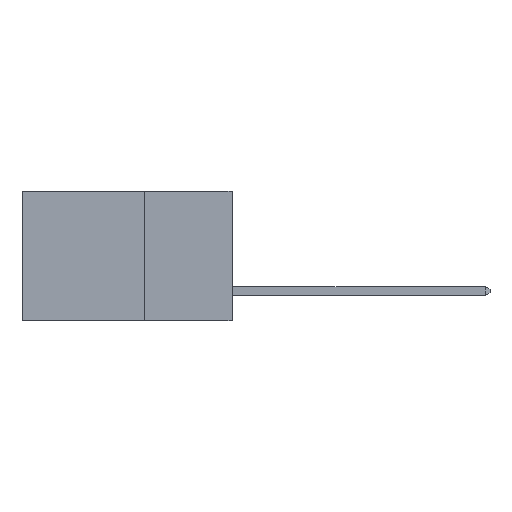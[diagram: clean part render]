
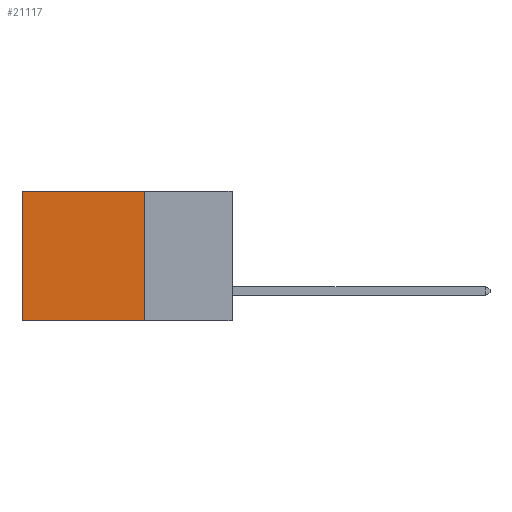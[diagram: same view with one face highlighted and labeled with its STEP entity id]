
A CAD part, left-side view. The second image highlights one B-rep face of the part: STEP entity #21117.
In plain terms, the highlighted planar face has unit normal (-1, 0, 0).
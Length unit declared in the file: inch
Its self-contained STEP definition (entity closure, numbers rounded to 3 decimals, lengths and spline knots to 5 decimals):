
#407 = VECTOR ( 'NONE', #17627, 39.37008 ) ;
#603 = DIRECTION ( 'NONE',  ( 0., 1., 0. ) ) ;
#798 = DIRECTION ( 'NONE',  ( 1., 0., 0. ) ) ;
#2346 = CARTESIAN_POINT ( 'NONE',  ( 0.2875, 0.25, 0. ) ) ;
#2445 = EDGE_CURVE ( 'NONE', #16082, #22579, #5867, .T. ) ;
#2901 = CARTESIAN_POINT ( 'NONE',  ( 0.2875, 0.6, 0. ) ) ;
#4182 = CARTESIAN_POINT ( 'NONE',  ( 0.2875, 0.6, -0.37 ) ) ;
#5738 = EDGE_CURVE ( 'NONE', #22579, #18657, #14520, .T. ) ;
#5787 = VECTOR ( 'NONE', #9420, 39.37008 ) ;
#5867 = LINE ( 'NONE', #2346, #14630 ) ;
#8053 = ORIENTED_EDGE ( 'NONE', *, *, #15060, .T. ) ;
#8632 = LINE ( 'NONE', #11225, #17955 ) ;
#9420 = DIRECTION ( 'NONE',  ( 0., 0., -1. ) ) ;
#10304 = CARTESIAN_POINT ( 'NONE',  ( 0.2875, 0.25, 0. ) ) ;
#10368 = ORIENTED_EDGE ( 'NONE', *, *, #19866, .T. ) ;
#10965 = VERTEX_POINT ( 'NONE', #2901 ) ;
#11225 = CARTESIAN_POINT ( 'NONE',  ( 0.2875, 0.25, 0. ) ) ;
#11958 = CARTESIAN_POINT ( 'NONE',  ( 0.2875, 0.25, -0.37 ) ) ;
#13042 = CARTESIAN_POINT ( 'NONE',  ( 0.2875, 0.6, 0. ) ) ;
#13188 = DIRECTION ( 'NONE',  ( 0., 0., -1. ) ) ;
#13786 = FACE_OUTER_BOUND ( 'NONE', #16669, .T. ) ;
#14038 = CARTESIAN_POINT ( 'NONE',  ( 0.2875, 0.25, -0.37 ) ) ;
#14520 = LINE ( 'NONE', #14038, #407 ) ;
#14630 = VECTOR ( 'NONE', #16441, 39.37008 ) ;
#15060 = EDGE_CURVE ( 'NONE', #10965, #18657, #19735, .T. ) ;
#16082 = VERTEX_POINT ( 'NONE', #10304 ) ;
#16441 = DIRECTION ( 'NONE',  ( 0., 0., -1. ) ) ;
#16669 = EDGE_LOOP ( 'NONE', ( #8053, #20697, #19980, #10368 ) ) ;
#17627 = DIRECTION ( 'NONE',  ( 0., 1., 0. ) ) ;
#17955 = VECTOR ( 'NONE', #603, 39.37008 ) ;
#18368 = CARTESIAN_POINT ( 'NONE',  ( 0.2875, 0.25, 0. ) ) ;
#18657 = VERTEX_POINT ( 'NONE', #4182 ) ;
#19735 = LINE ( 'NONE', #13042, #5787 ) ;
#19866 = EDGE_CURVE ( 'NONE', #16082, #10965, #8632, .T. ) ;
#19980 = ORIENTED_EDGE ( 'NONE', *, *, #2445, .F. ) ;
#20119 = PLANE ( 'NONE',  #21633 ) ;
#20697 = ORIENTED_EDGE ( 'NONE', *, *, #5738, .F. ) ;
#21117 = ADVANCED_FACE ( 'NONE', ( #13786 ), #20119, .F. ) ;
#21633 = AXIS2_PLACEMENT_3D ( 'NONE', #18368, #798, #13188 ) ;
#22579 = VERTEX_POINT ( 'NONE', #11958 ) ;
